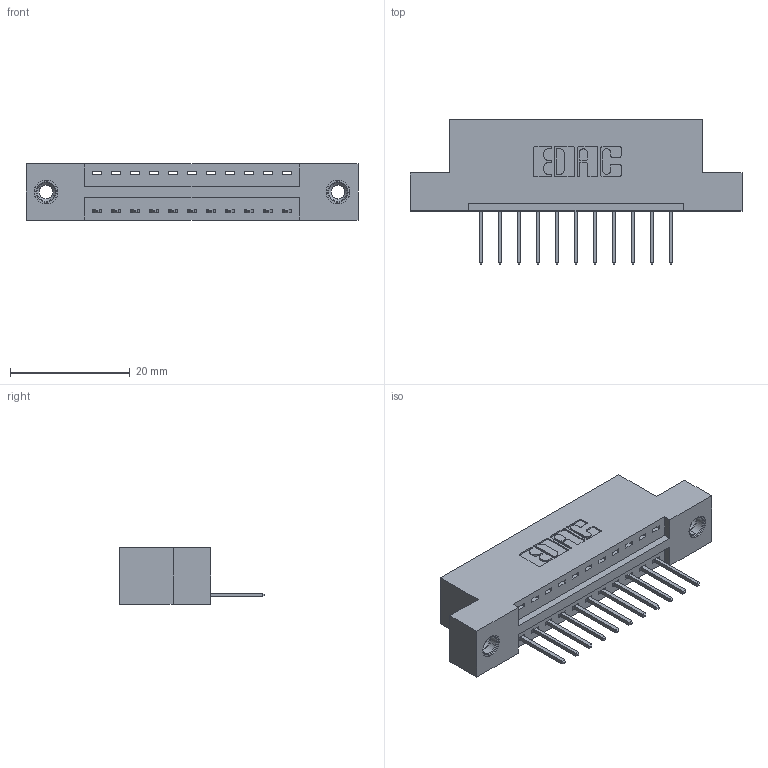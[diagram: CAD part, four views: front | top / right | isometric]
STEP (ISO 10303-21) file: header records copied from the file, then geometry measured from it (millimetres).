
FILE_DESCRIPTION (( 'STEP AP203' ), '1' );
FILE_NAME ('396-011-526-108.STEP', '2019-10-26T14:56:55', ( '' ), ( '' ), 'SwSTEP 2.0', 'SolidWorks 2016', '' );
FILE_SCHEMA (( 'CONFIG_CONTROL_DESIGN' ));
Length unit declared in the file: inch
Products named in the file (4): 396-011-526-108; 345-250-001_345-250-003-102; 346 Part_Flush Mounting Lugs - 0.156 Dia-TI; 345-292-001_345-293-126
Assembly tree (14 placements, depth 2):
  396-011-526-108
    346 Part_Flush Mounting Lugs - 0.156 Dia-TI
    345-292-001_345-293-126  x11
    345-250-001_345-250-003-102  x2
Bounding box: 55.5 x 24.13 x 9.4 mm (x, y, z)
Volume: 5083.6 mm3; surface area: 6030.4 mm2
Topology: 14 solids, 14 shells, 820 faces, 2401 edges, 1578 vertices
Faces by surface type: plane 548, cylinder 256, cone 12, torus 4
Entity records: 12204 total; most frequent: CARTESIAN_POINT 2084, ORIENTED_EDGE 2022, DIRECTION 1903, EDGE_CURVE 1011, VECTOR 815, LINE 815, VERTEX_POINT 668, AXIS2_PLACEMENT_3D 544
